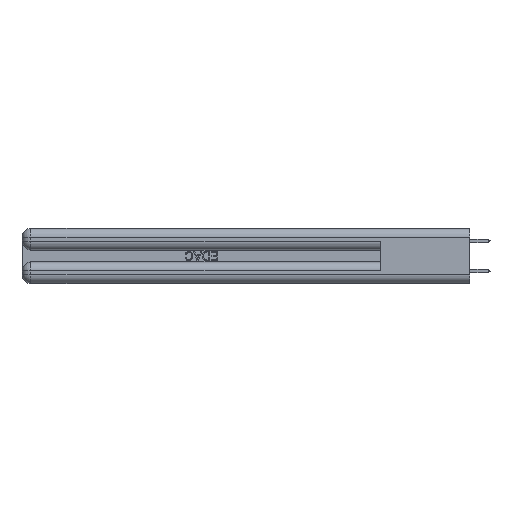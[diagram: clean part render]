
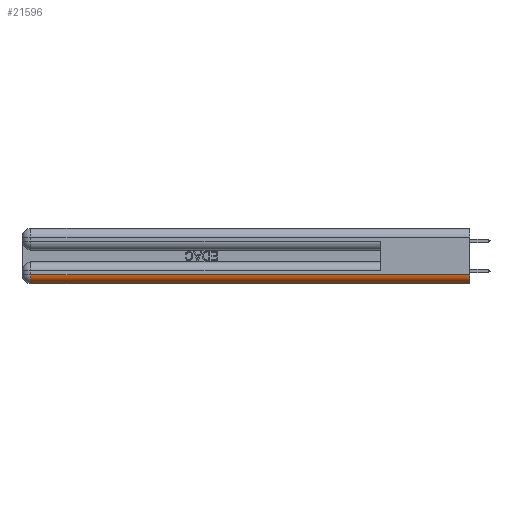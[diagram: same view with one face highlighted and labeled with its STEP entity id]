
A CAD part, left-side view. The second image highlights one B-rep face of the part: STEP entity #21596.
In plain terms, the highlighted cylindrical face has radius 1.524 mm (diameter 3.048 mm), a partial arc.
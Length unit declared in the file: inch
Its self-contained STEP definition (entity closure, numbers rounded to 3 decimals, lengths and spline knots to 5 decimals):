
#1698 = CARTESIAN_POINT ( 'NONE',  ( 0.06, 2.94, 0.06 ) ) ;
#2133 = AXIS2_PLACEMENT_3D ( 'NONE', #14942, #29698, #7108 ) ;
#5233 = CARTESIAN_POINT ( 'NONE',  ( 0.06, 3., 0. ) ) ;
#6700 = ORIENTED_EDGE ( 'NONE', *, *, #19217, .F. ) ;
#7108 = DIRECTION ( 'NONE',  ( 0., 0., 1. ) ) ;
#10863 = VERTEX_POINT ( 'NONE', #38066 ) ;
#11948 = CIRCLE ( 'NONE', #19309, 0.06 ) ;
#12667 = EDGE_CURVE ( 'NONE', #45258, #30937, #11948, .T. ) ;
#14244 = EDGE_CURVE ( 'NONE', #40816, #10863, #32374, .T. ) ;
#14942 = CARTESIAN_POINT ( 'NONE',  ( 0.06, 0., 0.06 ) ) ;
#16001 = DIRECTION ( 'NONE',  ( 0., 1., 0. ) ) ;
#16130 = CYLINDRICAL_SURFACE ( 'NONE', #2133, 0.06 ) ;
#17532 = CARTESIAN_POINT ( 'NONE',  ( 0., 0., 0.06 ) ) ;
#18556 = ORIENTED_EDGE ( 'NONE', *, *, #14244, .F. ) ;
#18945 = DIRECTION ( 'NONE',  ( 0., -1., 0. ) ) ;
#19217 = EDGE_CURVE ( 'NONE', #30937, #40816, #47419, .T. ) ;
#19309 = AXIS2_PLACEMENT_3D ( 'NONE', #1698, #27913, #24619 ) ;
#21596 = ADVANCED_FACE ( 'NONE', ( #24389 ), #16130, .T. ) ;
#24389 = FACE_OUTER_BOUND ( 'NONE', #43312, .T. ) ;
#24619 = DIRECTION ( 'NONE',  ( 0., 0., 1. ) ) ;
#25822 = ORIENTED_EDGE ( 'NONE', *, *, #29252, .F. ) ;
#26633 = VECTOR ( 'NONE', #16001, 39.37008 ) ;
#26645 = DIRECTION ( 'NONE',  ( 0., 0., 1. ) ) ;
#27913 = DIRECTION ( 'NONE',  ( 0., 1., 0. ) ) ;
#29252 = EDGE_CURVE ( 'NONE', #10863, #45258, #39451, .T. ) ;
#29512 = CARTESIAN_POINT ( 'NONE',  ( 0.06, 2.94, 0. ) ) ;
#29698 = DIRECTION ( 'NONE',  ( 0., 1., 0. ) ) ;
#30268 = ORIENTED_EDGE ( 'NONE', *, *, #12667, .F. ) ;
#30937 = VERTEX_POINT ( 'NONE', #39429 ) ;
#32374 = CIRCLE ( 'NONE', #36253, 0.06 ) ;
#33959 = CARTESIAN_POINT ( 'NONE',  ( 0.06, 0., 0.06 ) ) ;
#36253 = AXIS2_PLACEMENT_3D ( 'NONE', #33959, #41512, #26645 ) ;
#38066 = CARTESIAN_POINT ( 'NONE',  ( 0.06, 0., 0. ) ) ;
#39429 = CARTESIAN_POINT ( 'NONE',  ( 0., 2.94, 0.06 ) ) ;
#39451 = LINE ( 'NONE', #5233, #26633 ) ;
#40816 = VERTEX_POINT ( 'NONE', #17532 ) ;
#41512 = DIRECTION ( 'NONE',  ( 0., -1., 0. ) ) ;
#43312 = EDGE_LOOP ( 'NONE', ( #18556, #6700, #30268, #25822 ) ) ;
#43890 = VECTOR ( 'NONE', #18945, 39.37008 ) ;
#44696 = CARTESIAN_POINT ( 'NONE',  ( 0., 0., 0.06 ) ) ;
#45258 = VERTEX_POINT ( 'NONE', #29512 ) ;
#47419 = LINE ( 'NONE', #44696, #43890 ) ;
